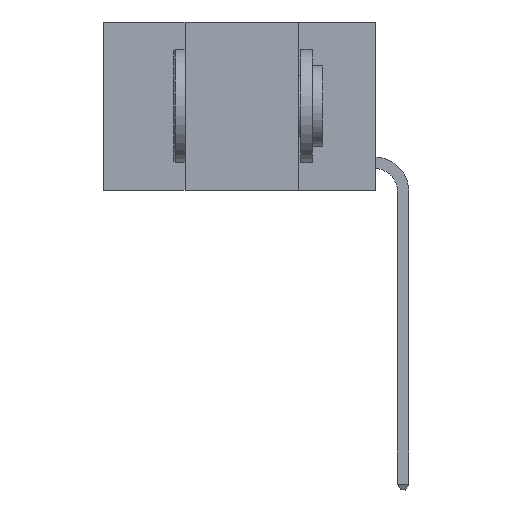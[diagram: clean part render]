
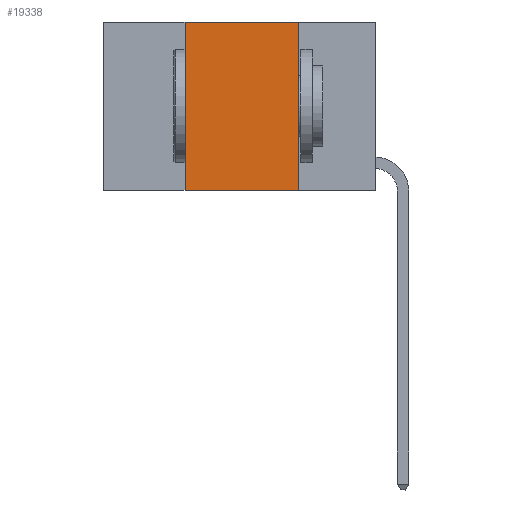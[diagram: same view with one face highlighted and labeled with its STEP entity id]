
A CAD part, left-side view. The second image highlights one B-rep face of the part: STEP entity #19338.
In plain terms, the highlighted planar face has unit normal (-1, 0, 0).
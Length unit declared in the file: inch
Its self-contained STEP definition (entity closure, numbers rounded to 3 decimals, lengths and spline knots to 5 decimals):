
#398 = DIRECTION ( 'NONE',  ( 0., -1., 0. ) ) ;
#1952 = EDGE_CURVE ( 'NONE', #2336, #14914, #19720, .T. ) ;
#2336 = VERTEX_POINT ( 'NONE', #21092 ) ;
#3084 = DIRECTION ( 'NONE',  ( 0., 0., 1. ) ) ;
#3358 = LINE ( 'NONE', #11811, #13578 ) ;
#3997 = LINE ( 'NONE', #4545, #24960 ) ;
#4472 = CARTESIAN_POINT ( 'NONE',  ( 0., 0.6, 0. ) ) ;
#4545 = CARTESIAN_POINT ( 'NONE',  ( 0., 0.6, -0.37 ) ) ;
#4590 = FACE_OUTER_BOUND ( 'NONE', #10842, .T. ) ;
#6630 = PLANE ( 'NONE',  #15300 ) ;
#10716 = DIRECTION ( 'NONE',  ( 0., 0., -1. ) ) ;
#10842 = EDGE_LOOP ( 'NONE', ( #17455, #17775, #20328, #20612 ) ) ;
#11276 = CARTESIAN_POINT ( 'NONE',  ( 0., 0.17, 0. ) ) ;
#11811 = CARTESIAN_POINT ( 'NONE',  ( 0., 0.17, 0. ) ) ;
#12671 = VECTOR ( 'NONE', #398, 39.37008 ) ;
#12750 = EDGE_CURVE ( 'NONE', #14914, #20186, #18098, .T. ) ;
#13201 = CARTESIAN_POINT ( 'NONE',  ( 0., 0.42, 0. ) ) ;
#13578 = VECTOR ( 'NONE', #13874, 39.37008 ) ;
#13874 = DIRECTION ( 'NONE',  ( 0., 0., -1. ) ) ;
#14776 = DIRECTION ( 'NONE',  ( 0., -1., 0. ) ) ;
#14914 = VERTEX_POINT ( 'NONE', #21779 ) ;
#15300 = AXIS2_PLACEMENT_3D ( 'NONE', #4472, #22879, #10716 ) ;
#17455 = ORIENTED_EDGE ( 'NONE', *, *, #24975, .F. ) ;
#17775 = ORIENTED_EDGE ( 'NONE', *, *, #12750, .F. ) ;
#18098 = LINE ( 'NONE', #24848, #12671 ) ;
#18156 = VERTEX_POINT ( 'NONE', #19656 ) ;
#19338 = ADVANCED_FACE ( 'NONE', ( #4590 ), #6630, .F. ) ;
#19656 = CARTESIAN_POINT ( 'NONE',  ( 0., 0.17, -0.37 ) ) ;
#19720 = LINE ( 'NONE', #13201, #24450 ) ;
#20186 = VERTEX_POINT ( 'NONE', #11276 ) ;
#20328 = ORIENTED_EDGE ( 'NONE', *, *, #1952, .F. ) ;
#20612 = ORIENTED_EDGE ( 'NONE', *, *, #26459, .T. ) ;
#21092 = CARTESIAN_POINT ( 'NONE',  ( 0., 0.42, -0.37 ) ) ;
#21779 = CARTESIAN_POINT ( 'NONE',  ( 0., 0.42, 0. ) ) ;
#22879 = DIRECTION ( 'NONE',  ( 1., 0., 0. ) ) ;
#24450 = VECTOR ( 'NONE', #3084, 39.37008 ) ;
#24848 = CARTESIAN_POINT ( 'NONE',  ( 0., 0.6, 0. ) ) ;
#24960 = VECTOR ( 'NONE', #14776, 39.37008 ) ;
#24975 = EDGE_CURVE ( 'NONE', #20186, #18156, #3358, .T. ) ;
#26459 = EDGE_CURVE ( 'NONE', #2336, #18156, #3997, .T. ) ;
